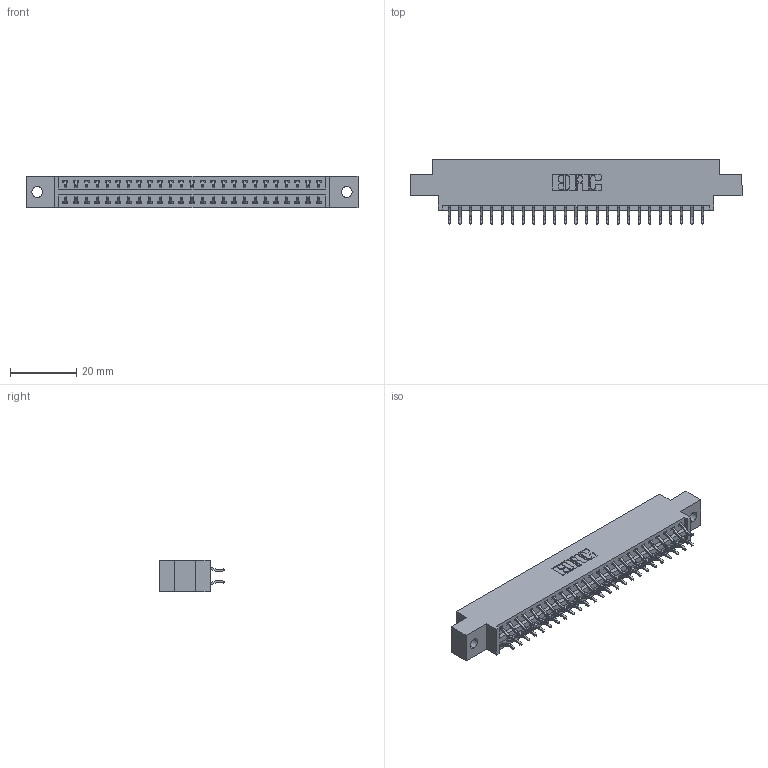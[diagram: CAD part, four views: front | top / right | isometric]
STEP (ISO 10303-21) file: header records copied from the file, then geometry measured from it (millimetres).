
FILE_DESCRIPTION (( 'STEP AP203' ), '1' );
FILE_NAME ('346-050-556-802.STEP', '2022-05-20T23:47:58', ( '' ), ( '' ), 'SwSTEP 2.0', 'SolidWorks 2020', '' );
FILE_SCHEMA (( 'CONFIG_CONTROL_DESIGN' ));
Length unit declared in the file: inch
Products named in the file (3): 346-050-556-802; 346 Part_0.170 Offset - 0.128 Dia; 345-292-001_556 Tail
Assembly tree (51 placements, depth 2):
  346-050-556-802
    346 Part_0.170 Offset - 0.128 Dia
    345-292-001_556 Tail  x50
Bounding box: 99.95 x 19.57 x 9.4 mm (x, y, z)
Volume: 9421 mm3; surface area: 12546.5 mm2
Topology: 51 solids, 51 shells, 3026 faces, 8991 edges, 5926 vertices
Faces by surface type: plane 2030, cylinder 996
Entity records: 18959 total; most frequent: CARTESIAN_POINT 3164, ORIENTED_EDGE 3086, DIRECTION 2827, EDGE_CURVE 1543, LINE 1303, VECTOR 1303, VERTEX_POINT 1026, AXIS2_PLACEMENT_3D 762
